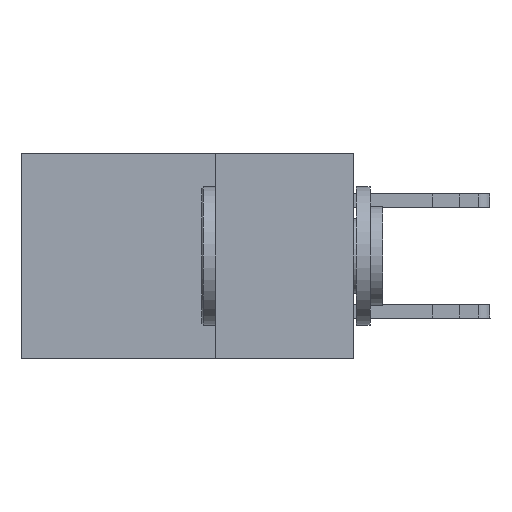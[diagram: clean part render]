
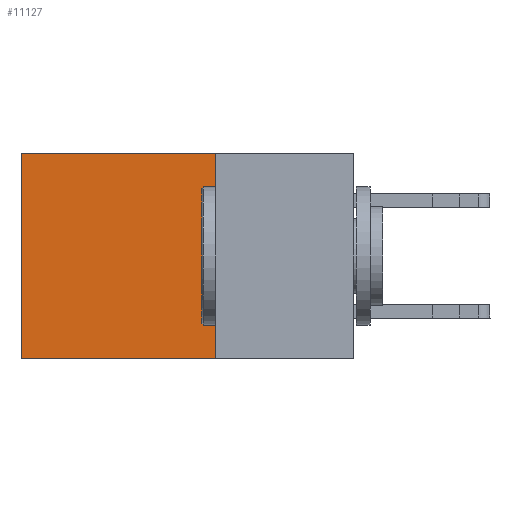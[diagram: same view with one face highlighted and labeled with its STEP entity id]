
A CAD part, left-side view. The second image highlights one B-rep face of the part: STEP entity #11127.
In plain terms, the highlighted planar face has unit normal (-1, 0, 0).
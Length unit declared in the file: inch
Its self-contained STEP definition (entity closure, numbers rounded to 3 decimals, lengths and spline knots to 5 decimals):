
#972 = LINE ( 'NONE', #7029, #26609 ) ;
#2512 = LINE ( 'NONE', #29460, #8378 ) ;
#5021 = LINE ( 'NONE', #9127, #33592 ) ;
#6923 = FACE_OUTER_BOUND ( 'NONE', #20626, .T. ) ;
#7029 = CARTESIAN_POINT ( 'NONE',  ( 0.2875, 0.25, 0. ) ) ;
#7673 = DIRECTION ( 'NONE',  ( 0., 0., -1. ) ) ;
#8235 = EDGE_CURVE ( 'NONE', #34089, #21111, #5021, .T. ) ;
#8378 = VECTOR ( 'NONE', #7673, 39.37008 ) ;
#9127 = CARTESIAN_POINT ( 'NONE',  ( 0.2875, 0.25, 0. ) ) ;
#11127 = ADVANCED_FACE ( 'NONE', ( #6923 ), #30248, .F. ) ;
#11490 = VERTEX_POINT ( 'NONE', #16264 ) ;
#14044 = DIRECTION ( 'NONE',  ( 0., 0., -1. ) ) ;
#14998 = DIRECTION ( 'NONE',  ( 0., 0., -1. ) ) ;
#16264 = CARTESIAN_POINT ( 'NONE',  ( 0.2875, 0.25, -0.37 ) ) ;
#16624 = CARTESIAN_POINT ( 'NONE',  ( 0.2875, 0.25, 0. ) ) ;
#20626 = EDGE_LOOP ( 'NONE', ( #21720, #22044, #30297, #27199 ) ) ;
#21111 = VERTEX_POINT ( 'NONE', #26104 ) ;
#21720 = ORIENTED_EDGE ( 'NONE', *, *, #32373, .T. ) ;
#22044 = ORIENTED_EDGE ( 'NONE', *, *, #24581, .F. ) ;
#23082 = LINE ( 'NONE', #26546, #26875 ) ;
#24581 = EDGE_CURVE ( 'NONE', #11490, #33371, #23082, .T. ) ;
#25555 = DIRECTION ( 'NONE',  ( 0., 1., 0. ) ) ;
#26104 = CARTESIAN_POINT ( 'NONE',  ( 0.2875, 0.6, 0. ) ) ;
#26420 = DIRECTION ( 'NONE',  ( 0., 1., 0. ) ) ;
#26546 = CARTESIAN_POINT ( 'NONE',  ( 0.2875, 0.25, -0.37 ) ) ;
#26609 = VECTOR ( 'NONE', #14998, 39.37008 ) ;
#26875 = VECTOR ( 'NONE', #26420, 39.37008 ) ;
#27199 = ORIENTED_EDGE ( 'NONE', *, *, #8235, .T. ) ;
#28327 = CARTESIAN_POINT ( 'NONE',  ( 0.2875, 0.6, -0.37 ) ) ;
#29460 = CARTESIAN_POINT ( 'NONE',  ( 0.2875, 0.6, 0. ) ) ;
#30248 = PLANE ( 'NONE',  #33514 ) ;
#30297 = ORIENTED_EDGE ( 'NONE', *, *, #32121, .F. ) ;
#32121 = EDGE_CURVE ( 'NONE', #34089, #11490, #972, .T. ) ;
#32373 = EDGE_CURVE ( 'NONE', #21111, #33371, #2512, .T. ) ;
#32648 = DIRECTION ( 'NONE',  ( 1., 0., 0. ) ) ;
#32797 = CARTESIAN_POINT ( 'NONE',  ( 0.2875, 0.25, 0. ) ) ;
#33371 = VERTEX_POINT ( 'NONE', #28327 ) ;
#33514 = AXIS2_PLACEMENT_3D ( 'NONE', #16624, #32648, #14044 ) ;
#33592 = VECTOR ( 'NONE', #25555, 39.37008 ) ;
#34089 = VERTEX_POINT ( 'NONE', #32797 ) ;
